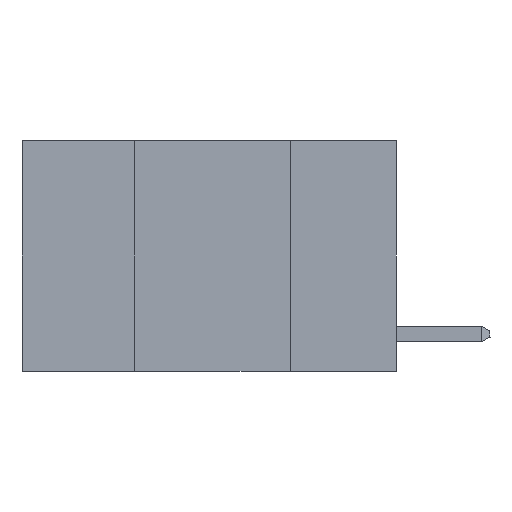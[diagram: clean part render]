
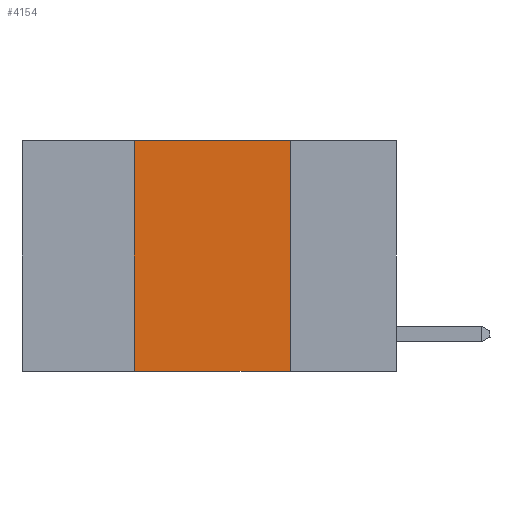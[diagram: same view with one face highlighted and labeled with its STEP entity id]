
A CAD part, left-side view. The second image highlights one B-rep face of the part: STEP entity #4154.
In plain terms, the highlighted planar face has unit normal (-1, 0, 0).
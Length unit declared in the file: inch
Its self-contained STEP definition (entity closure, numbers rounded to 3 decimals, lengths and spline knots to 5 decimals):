
#667 = FACE_OUTER_BOUND ( 'NONE', #16725, .T. ) ;
#1059 = ORIENTED_EDGE ( 'NONE', *, *, #9328, .T. ) ;
#1728 = DIRECTION ( 'NONE',  ( 0., -1., 0. ) ) ;
#2117 = LINE ( 'NONE', #15868, #10123 ) ;
#2342 = DIRECTION ( 'NONE',  ( 1., 0., 0. ) ) ;
#2347 = VECTOR ( 'NONE', #10646, 39.37008 ) ;
#3206 = VERTEX_POINT ( 'NONE', #21568 ) ;
#4154 = ADVANCED_FACE ( 'NONE', ( #667 ), #19130, .F. ) ;
#4240 = EDGE_CURVE ( 'NONE', #10282, #18150, #7851, .T. ) ;
#4617 = AXIS2_PLACEMENT_3D ( 'NONE', #17339, #2342, #20931 ) ;
#4872 = ORIENTED_EDGE ( 'NONE', *, *, #20647, .F. ) ;
#5461 = LINE ( 'NONE', #20663, #2347 ) ;
#5541 = LINE ( 'NONE', #8923, #20550 ) ;
#6638 = CARTESIAN_POINT ( 'NONE',  ( 0., 0.42, 0. ) ) ;
#7344 = CARTESIAN_POINT ( 'NONE',  ( 0., 0.42, -0.37 ) ) ;
#7851 = LINE ( 'NONE', #7968, #21172 ) ;
#7968 = CARTESIAN_POINT ( 'NONE',  ( 0., 0.42, 0. ) ) ;
#8899 = ORIENTED_EDGE ( 'NONE', *, *, #4240, .F. ) ;
#8923 = CARTESIAN_POINT ( 'NONE',  ( 0., 0.6, 0. ) ) ;
#9328 = EDGE_CURVE ( 'NONE', #10282, #3206, #2117, .T. ) ;
#10123 = VECTOR ( 'NONE', #14063, 39.37008 ) ;
#10282 = VERTEX_POINT ( 'NONE', #7344 ) ;
#10646 = DIRECTION ( 'NONE',  ( 0., 0., -1. ) ) ;
#11461 = DIRECTION ( 'NONE',  ( 0., 0., 1. ) ) ;
#12583 = CARTESIAN_POINT ( 'NONE',  ( 0., 0.17, 0. ) ) ;
#13118 = EDGE_CURVE ( 'NONE', #18150, #15432, #5541, .T. ) ;
#14063 = DIRECTION ( 'NONE',  ( 0., -1., 0. ) ) ;
#15432 = VERTEX_POINT ( 'NONE', #12583 ) ;
#15868 = CARTESIAN_POINT ( 'NONE',  ( 0., 0.6, -0.37 ) ) ;
#16670 = ORIENTED_EDGE ( 'NONE', *, *, #13118, .F. ) ;
#16725 = EDGE_LOOP ( 'NONE', ( #4872, #16670, #8899, #1059 ) ) ;
#17339 = CARTESIAN_POINT ( 'NONE',  ( 0., 0.6, 0. ) ) ;
#18150 = VERTEX_POINT ( 'NONE', #6638 ) ;
#19130 = PLANE ( 'NONE',  #4617 ) ;
#20550 = VECTOR ( 'NONE', #1728, 39.37008 ) ;
#20647 = EDGE_CURVE ( 'NONE', #15432, #3206, #5461, .T. ) ;
#20663 = CARTESIAN_POINT ( 'NONE',  ( 0., 0.17, 0. ) ) ;
#20931 = DIRECTION ( 'NONE',  ( 0., 0., -1. ) ) ;
#21172 = VECTOR ( 'NONE', #11461, 39.37008 ) ;
#21568 = CARTESIAN_POINT ( 'NONE',  ( 0., 0.17, -0.37 ) ) ;
